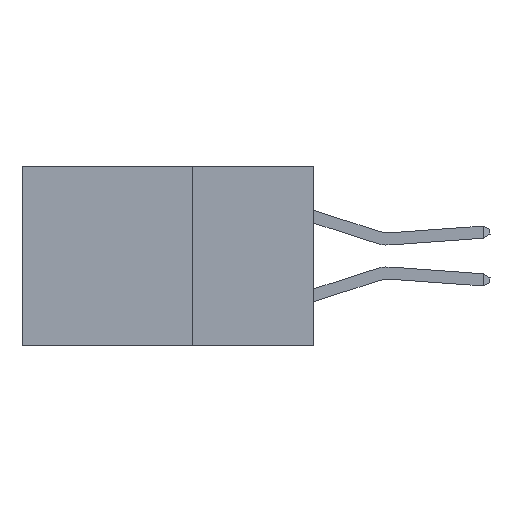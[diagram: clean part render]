
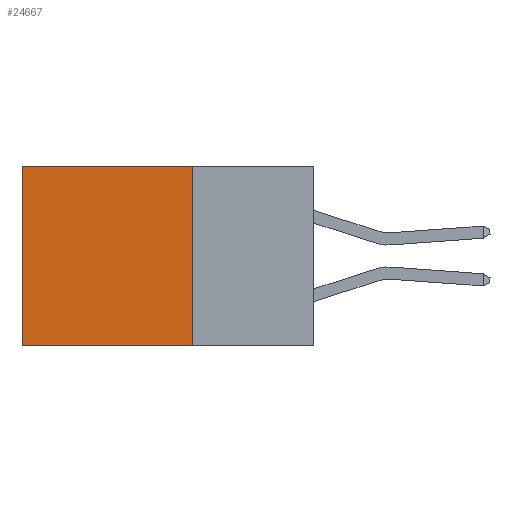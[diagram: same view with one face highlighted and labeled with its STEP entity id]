
A CAD part, left-side view. The second image highlights one B-rep face of the part: STEP entity #24667.
In plain terms, the highlighted planar face has unit normal (-1, 0, 0).
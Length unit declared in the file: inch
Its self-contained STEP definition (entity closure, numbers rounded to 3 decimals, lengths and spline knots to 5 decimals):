
#569 = LINE ( 'NONE', #15596, #21847 ) ;
#662 = VECTOR ( 'NONE', #6231, 39.37008 ) ;
#730 = EDGE_CURVE ( 'NONE', #27212, #18280, #26067, .T. ) ;
#1674 = LINE ( 'NONE', #2334, #27368 ) ;
#2334 = CARTESIAN_POINT ( 'NONE',  ( 0.2875, 0.25, -0.37 ) ) ;
#2495 = VECTOR ( 'NONE', #3957, 39.37008 ) ;
#3957 = DIRECTION ( 'NONE',  ( 0., 1., 0. ) ) ;
#4619 = CARTESIAN_POINT ( 'NONE',  ( 0.2875, 0.25, -0.37 ) ) ;
#5008 = EDGE_LOOP ( 'NONE', ( #27562, #9019, #15086, #19793 ) ) ;
#5088 = PLANE ( 'NONE',  #18454 ) ;
#5181 = CARTESIAN_POINT ( 'NONE',  ( 0.2875, 0.25, 0. ) ) ;
#6133 = CARTESIAN_POINT ( 'NONE',  ( 0.2875, 0.25, 0. ) ) ;
#6231 = DIRECTION ( 'NONE',  ( 0., 0., -1. ) ) ;
#7268 = DIRECTION ( 'NONE',  ( 0., 0., -1. ) ) ;
#7465 = DIRECTION ( 'NONE',  ( 1., 0., 0. ) ) ;
#8002 = LINE ( 'NONE', #23279, #2495 ) ;
#8798 = VERTEX_POINT ( 'NONE', #9015 ) ;
#9015 = CARTESIAN_POINT ( 'NONE',  ( 0.2875, 0.6, -0.37 ) ) ;
#9019 = ORIENTED_EDGE ( 'NONE', *, *, #17438, .F. ) ;
#9826 = CARTESIAN_POINT ( 'NONE',  ( 0.2875, 0.6, 0. ) ) ;
#11718 = CARTESIAN_POINT ( 'NONE',  ( 0.2875, 0.25, 0. ) ) ;
#15026 = FACE_OUTER_BOUND ( 'NONE', #5008, .T. ) ;
#15086 = ORIENTED_EDGE ( 'NONE', *, *, #730, .F. ) ;
#15596 = CARTESIAN_POINT ( 'NONE',  ( 0.2875, 0.6, 0. ) ) ;
#17438 = EDGE_CURVE ( 'NONE', #18280, #8798, #1674, .T. ) ;
#17738 = DIRECTION ( 'NONE',  ( 0., 0., -1. ) ) ;
#18211 = EDGE_CURVE ( 'NONE', #25363, #8798, #569, .T. ) ;
#18280 = VERTEX_POINT ( 'NONE', #4619 ) ;
#18454 = AXIS2_PLACEMENT_3D ( 'NONE', #5181, #7465, #7268 ) ;
#19793 = ORIENTED_EDGE ( 'NONE', *, *, #21332, .T. ) ;
#21332 = EDGE_CURVE ( 'NONE', #27212, #25363, #8002, .T. ) ;
#21847 = VECTOR ( 'NONE', #17738, 39.37008 ) ;
#23279 = CARTESIAN_POINT ( 'NONE',  ( 0.2875, 0.25, 0. ) ) ;
#24667 = ADVANCED_FACE ( 'NONE', ( #15026 ), #5088, .F. ) ;
#25363 = VERTEX_POINT ( 'NONE', #9826 ) ;
#26067 = LINE ( 'NONE', #6133, #662 ) ;
#26288 = DIRECTION ( 'NONE',  ( 0., 1., 0. ) ) ;
#27212 = VERTEX_POINT ( 'NONE', #11718 ) ;
#27368 = VECTOR ( 'NONE', #26288, 39.37008 ) ;
#27562 = ORIENTED_EDGE ( 'NONE', *, *, #18211, .T. ) ;
